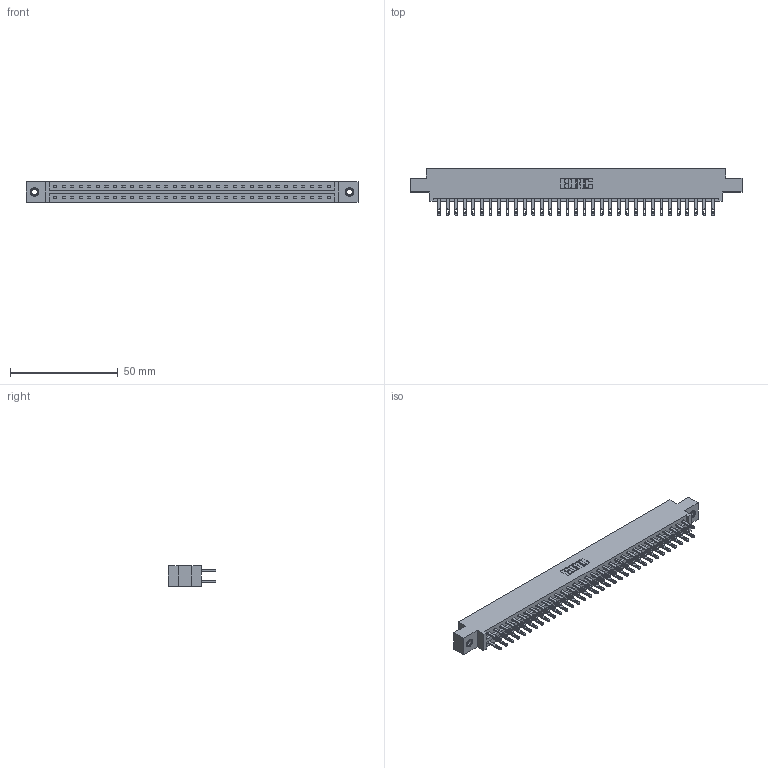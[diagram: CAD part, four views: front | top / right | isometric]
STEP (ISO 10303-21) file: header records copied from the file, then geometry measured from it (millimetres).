
FILE_DESCRIPTION (( 'STEP AP203' ), '1' );
FILE_NAME ('337-066-500-807.STEP', '2019-10-12T00:29:26', ( '' ), ( '' ), 'SwSTEP 2.0', 'SolidWorks 2016', '' );
FILE_SCHEMA (( 'CONFIG_CONTROL_DESIGN' ));
Length unit declared in the file: inch
Products named in the file (4): 337-066-500-807; 345-250-001_345-250-005-103; 337 Part_0.170 Offset - 0.156 Dia-TI; 345-292-001_345-293-100
Assembly tree (69 placements, depth 2):
  337-066-500-807
    337 Part_0.170 Offset - 0.156 Dia-TI
    345-292-001_345-293-100  x66
    345-250-001_345-250-005-103  x2
Bounding box: 153.77 x 21.85 x 9.4 mm (x, y, z)
Volume: 16156.5 mm3; surface area: 19053.7 mm2
Topology: 69 solids, 69 shells, 3478 faces, 10557 edges, 7030 vertices
Faces by surface type: plane 2218, cylinder 1244, cone 12, torus 4
Entity records: 27998 total; most frequent: CARTESIAN_POINT 4705, ORIENTED_EDGE 4634, DIRECTION 4051, EDGE_CURVE 2317, VECTOR 2165, LINE 2165, VERTEX_POINT 1540, AXIS2_PLACEMENT_3D 943
